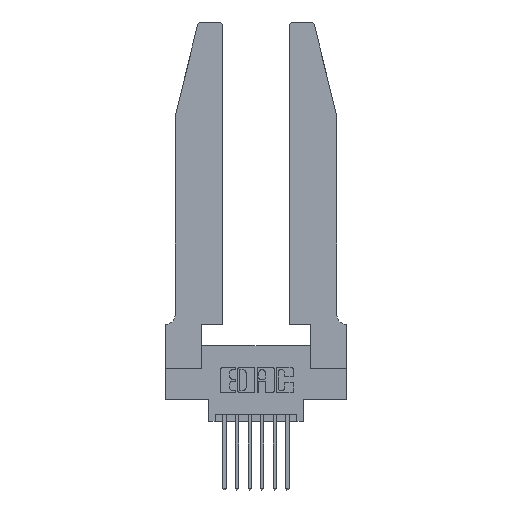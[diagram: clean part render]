
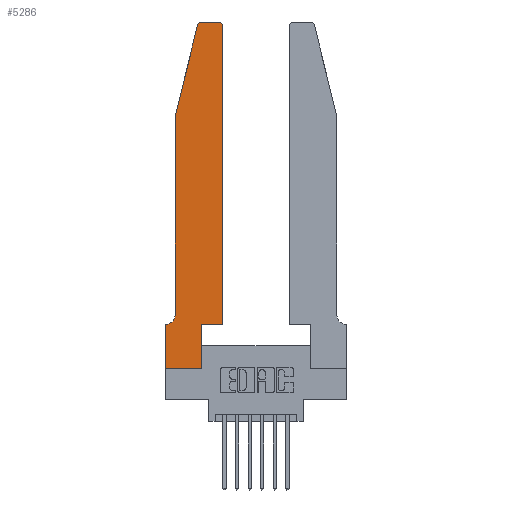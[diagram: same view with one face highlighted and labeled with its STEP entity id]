
A CAD part, top view. The second image highlights one B-rep face of the part: STEP entity #5286.
In plain terms, the highlighted planar face has unit normal (0, 0, 1).
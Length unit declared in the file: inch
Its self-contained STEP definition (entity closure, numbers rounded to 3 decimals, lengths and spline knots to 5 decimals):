
#127 = VERTEX_POINT ( 'NONE', #4604 ) ;
#276 = VECTOR ( 'NONE', #6572, 39.37008 ) ;
#405 = CARTESIAN_POINT ( 'NONE',  ( 0.284, 2.72, 0.37 ) ) ;
#595 = ORIENTED_EDGE ( 'NONE', *, *, #3409, .T. ) ;
#605 = CARTESIAN_POINT ( 'NONE',  ( 0.0755, 0.35, 0.37 ) ) ;
#613 = CARTESIAN_POINT ( 'NONE',  ( 0., 0., 0.37 ) ) ;
#796 = LINE ( 'NONE', #11033, #276 ) ;
#882 = CARTESIAN_POINT ( 'NONE',  ( 0., 0.35, 0.37 ) ) ;
#917 = EDGE_CURVE ( 'NONE', #9800, #3431, #12850, .T. ) ;
#1035 = VECTOR ( 'NONE', #8098, 39.37008 ) ;
#1044 = CARTESIAN_POINT ( 'NONE',  ( 0., 0., 0.37 ) ) ;
#1154 = CIRCLE ( 'NONE', #8791, 0.03 ) ;
#1281 = ORIENTED_EDGE ( 'NONE', *, *, #11400, .T. ) ;
#1288 = CARTESIAN_POINT ( 'NONE',  ( 0.0055, 0.35, 0.37 ) ) ;
#1332 = VERTEX_POINT ( 'NONE', #8363 ) ;
#1445 = CARTESIAN_POINT ( 'NONE',  ( 0.4505, 0.35, 0.37 ) ) ;
#1532 = EDGE_CURVE ( 'NONE', #1332, #2453, #796, .T. ) ;
#1557 = DIRECTION ( 'NONE',  ( 0., 0., 1. ) ) ;
#1702 = ORIENTED_EDGE ( 'NONE', *, *, #10204, .T. ) ;
#2071 = CARTESIAN_POINT ( 'NONE',  ( 0.284, 2.75, 0.37 ) ) ;
#2187 = ORIENTED_EDGE ( 'NONE', *, *, #9994, .T. ) ;
#2387 = LINE ( 'NONE', #1445, #12041 ) ;
#2453 = VERTEX_POINT ( 'NONE', #2071 ) ;
#2457 = AXIS2_PLACEMENT_3D ( 'NONE', #13019, #6284, #6851 ) ;
#2527 = CARTESIAN_POINT ( 'NONE',  ( 0.2865, 0.35, 0.37 ) ) ;
#2802 = CIRCLE ( 'NONE', #11562, 0.03 ) ;
#2815 = VECTOR ( 'NONE', #10329, 39.37008 ) ;
#2915 = EDGE_CURVE ( 'NONE', #3431, #7545, #2995, .T. ) ;
#2995 = LINE ( 'NONE', #2527, #2815 ) ;
#3409 = EDGE_CURVE ( 'NONE', #10399, #4732, #8906, .T. ) ;
#3431 = VERTEX_POINT ( 'NONE', #10273 ) ;
#3619 = ORIENTED_EDGE ( 'NONE', *, *, #7117, .T. ) ;
#3853 = DIRECTION ( 'NONE',  ( 0., 0., 1. ) ) ;
#4318 = VERTEX_POINT ( 'NONE', #11209 ) ;
#4325 = ORIENTED_EDGE ( 'NONE', *, *, #917, .T. ) ;
#4604 = CARTESIAN_POINT ( 'NONE',  ( 0.25487, 2.72718, 0.37 ) ) ;
#4732 = VERTEX_POINT ( 'NONE', #9540 ) ;
#4842 = DIRECTION ( 'NONE',  ( 0., 1., 0. ) ) ;
#5063 = VECTOR ( 'NONE', #8087, 39.37008 ) ;
#5105 = DIRECTION ( 'NONE',  ( 1., 0., 0. ) ) ;
#5256 = ORIENTED_EDGE ( 'NONE', *, *, #9562, .T. ) ;
#5286 = ADVANCED_FACE ( 'NONE', ( #7775 ), #12336, .T. ) ;
#5360 = EDGE_CURVE ( 'NONE', #4318, #9625, #2387, .T. ) ;
#5492 = CARTESIAN_POINT ( 'NONE',  ( 0.4505, 0.35, 0.37 ) ) ;
#5764 = ORIENTED_EDGE ( 'NONE', *, *, #6941, .T. ) ;
#5928 = VECTOR ( 'NONE', #10413, 39.37008 ) ;
#6037 = VECTOR ( 'NONE', #6267, 39.37008 ) ;
#6102 = CARTESIAN_POINT ( 'NONE',  ( 0.0755, 2., 0.37 ) ) ;
#6202 = CARTESIAN_POINT ( 'NONE',  ( 0.4205, 2.72, 0.37 ) ) ;
#6267 = DIRECTION ( 'NONE',  ( -1., 0., 0. ) ) ;
#6284 = DIRECTION ( 'NONE',  ( 0., 0., -1. ) ) ;
#6572 = DIRECTION ( 'NONE',  ( -1., 0., 0. ) ) ;
#6851 = DIRECTION ( 'NONE',  ( -1., 0., 0. ) ) ;
#6941 = EDGE_CURVE ( 'NONE', #9761, #10769, #13427, .T. ) ;
#6949 = DIRECTION ( 'NONE',  ( 1., 0., 0. ) ) ;
#7117 = EDGE_CURVE ( 'NONE', #2453, #127, #1154, .T. ) ;
#7284 = EDGE_LOOP ( 'NONE', ( #10495, #3619, #1281, #595, #13102, #5764, #1702, #4325, #13909, #5256, #8178, #2187 ) ) ;
#7384 = DIRECTION ( 'NONE',  ( 1., 0., 0. ) ) ;
#7545 = VERTEX_POINT ( 'NONE', #8172 ) ;
#7640 = AXIS2_PLACEMENT_3D ( 'NONE', #14487, #11202, #7647 ) ;
#7647 = DIRECTION ( 'NONE',  ( 1., 0., 0. ) ) ;
#7662 = LINE ( 'NONE', #5492, #9428 ) ;
#7775 = FACE_OUTER_BOUND ( 'NONE', #7284, .T. ) ;
#8087 = DIRECTION ( 'NONE',  ( 0., -1., 0. ) ) ;
#8098 = DIRECTION ( 'NONE',  ( -0.239, -0.971, 0. ) ) ;
#8172 = CARTESIAN_POINT ( 'NONE',  ( 0.2865, 0.35, 0.37 ) ) ;
#8178 = ORIENTED_EDGE ( 'NONE', *, *, #5360, .T. ) ;
#8363 = CARTESIAN_POINT ( 'NONE',  ( 0.4205, 2.75, 0.37 ) ) ;
#8416 = EDGE_CURVE ( 'NONE', #4732, #9761, #8933, .T. ) ;
#8791 = AXIS2_PLACEMENT_3D ( 'NONE', #405, #1557, #6949 ) ;
#8906 = LINE ( 'NONE', #12657, #5928 ) ;
#8933 = CIRCLE ( 'NONE', #2457, 0.07 ) ;
#9428 = VECTOR ( 'NONE', #13310, 39.37008 ) ;
#9540 = CARTESIAN_POINT ( 'NONE',  ( 0.0755, 0.42, 0.37 ) ) ;
#9562 = EDGE_CURVE ( 'NONE', #7545, #4318, #7662, .T. ) ;
#9625 = VERTEX_POINT ( 'NONE', #10977 ) ;
#9761 = VERTEX_POINT ( 'NONE', #1288 ) ;
#9800 = VERTEX_POINT ( 'NONE', #1044 ) ;
#9994 = EDGE_CURVE ( 'NONE', #9625, #1332, #2802, .T. ) ;
#10204 = EDGE_CURVE ( 'NONE', #10769, #9800, #13828, .T. ) ;
#10246 = LINE ( 'NONE', #6102, #1035 ) ;
#10273 = CARTESIAN_POINT ( 'NONE',  ( 0.2865, 0., 0.37 ) ) ;
#10329 = DIRECTION ( 'NONE',  ( 0., 1., 0. ) ) ;
#10399 = VERTEX_POINT ( 'NONE', #13023 ) ;
#10413 = DIRECTION ( 'NONE',  ( 0., -1., 0. ) ) ;
#10495 = ORIENTED_EDGE ( 'NONE', *, *, #1532, .T. ) ;
#10769 = VERTEX_POINT ( 'NONE', #882 ) ;
#10977 = CARTESIAN_POINT ( 'NONE',  ( 0.4505, 2.72, 0.37 ) ) ;
#11033 = CARTESIAN_POINT ( 'NONE',  ( 0.2605, 2.75, 0.37 ) ) ;
#11071 = VECTOR ( 'NONE', #7384, 39.37008 ) ;
#11202 = DIRECTION ( 'NONE',  ( 0., 0., 1. ) ) ;
#11209 = CARTESIAN_POINT ( 'NONE',  ( 0.4505, 0.35, 0.37 ) ) ;
#11400 = EDGE_CURVE ( 'NONE', #127, #10399, #10246, .T. ) ;
#11562 = AXIS2_PLACEMENT_3D ( 'NONE', #6202, #3853, #5105 ) ;
#12041 = VECTOR ( 'NONE', #4842, 39.37008 ) ;
#12336 = PLANE ( 'NONE',  #7640 ) ;
#12657 = CARTESIAN_POINT ( 'NONE',  ( 0.0755, 2., 0.37 ) ) ;
#12850 = LINE ( 'NONE', #613, #11071 ) ;
#13019 = CARTESIAN_POINT ( 'NONE',  ( 0.0055, 0.42, 0.37 ) ) ;
#13023 = CARTESIAN_POINT ( 'NONE',  ( 0.0755, 2., 0.37 ) ) ;
#13102 = ORIENTED_EDGE ( 'NONE', *, *, #8416, .T. ) ;
#13310 = DIRECTION ( 'NONE',  ( 1., 0., 0. ) ) ;
#13427 = LINE ( 'NONE', #605, #6037 ) ;
#13828 = LINE ( 'NONE', #13860, #5063 ) ;
#13860 = CARTESIAN_POINT ( 'NONE',  ( 0., 0., 0.37 ) ) ;
#13909 = ORIENTED_EDGE ( 'NONE', *, *, #2915, .T. ) ;
#14487 = CARTESIAN_POINT ( 'NONE',  ( 0., 0.35, 0.37 ) ) ;
